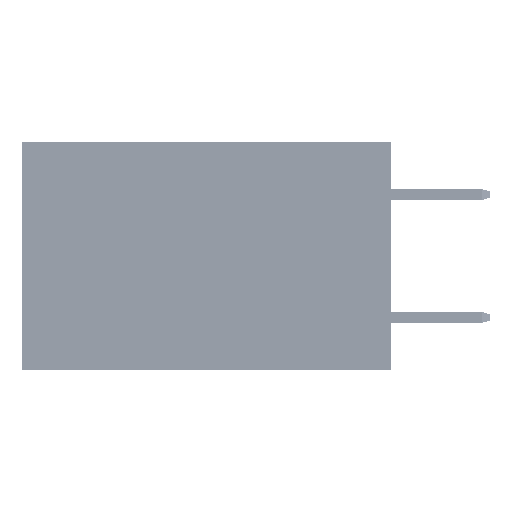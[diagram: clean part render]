
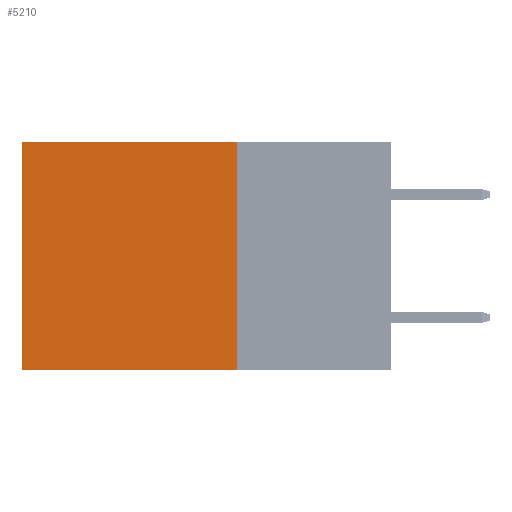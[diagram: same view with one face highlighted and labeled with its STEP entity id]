
A CAD part, left-side view. The second image highlights one B-rep face of the part: STEP entity #5210.
In plain terms, the highlighted planar face has unit normal (-1, 0, 0).
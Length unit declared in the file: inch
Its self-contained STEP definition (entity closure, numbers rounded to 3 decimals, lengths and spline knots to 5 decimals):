
#3151 = CARTESIAN_POINT ( 'NONE',  ( 0.2875, 0.25, 0. ) ) ;
#4904 = VECTOR ( 'NONE', #6634, 39.37008 ) ;
#5210 = ADVANCED_FACE ( 'NONE', ( #14518 ), #25948, .F. ) ;
#5528 = ORIENTED_EDGE ( 'NONE', *, *, #47186, .T. ) ;
#6573 = ORIENTED_EDGE ( 'NONE', *, *, #26342, .F. ) ;
#6634 = DIRECTION ( 'NONE',  ( 0., 1., 0. ) ) ;
#7434 = VERTEX_POINT ( 'NONE', #32129 ) ;
#8522 = VECTOR ( 'NONE', #39454, 39.37008 ) ;
#9106 = ORIENTED_EDGE ( 'NONE', *, *, #10187, .F. ) ;
#9774 = VECTOR ( 'NONE', #40423, 39.37008 ) ;
#10187 = EDGE_CURVE ( 'NONE', #12252, #39724, #34693, .T. ) ;
#10307 = EDGE_CURVE ( 'NONE', #17589, #7434, #33476, .T. ) ;
#12252 = VERTEX_POINT ( 'NONE', #25868 ) ;
#12805 = LINE ( 'NONE', #33045, #9774 ) ;
#14476 = DIRECTION ( 'NONE',  ( 1., 0., 0. ) ) ;
#14518 = FACE_OUTER_BOUND ( 'NONE', #28365, .T. ) ;
#17578 = CARTESIAN_POINT ( 'NONE',  ( 0.2875, 0.25, 0. ) ) ;
#17589 = VERTEX_POINT ( 'NONE', #31021 ) ;
#25868 = CARTESIAN_POINT ( 'NONE',  ( 0.2875, 0.25, -0.37 ) ) ;
#25948 = PLANE ( 'NONE',  #30757 ) ;
#26342 = EDGE_CURVE ( 'NONE', #17589, #12252, #12805, .T. ) ;
#26993 = ORIENTED_EDGE ( 'NONE', *, *, #10307, .T. ) ;
#28257 = CARTESIAN_POINT ( 'NONE',  ( 0.2875, 0.6, -0.37 ) ) ;
#28365 = EDGE_LOOP ( 'NONE', ( #5528, #9106, #6573, #26993 ) ) ;
#29901 = DIRECTION ( 'NONE',  ( 0., 0., -1. ) ) ;
#30757 = AXIS2_PLACEMENT_3D ( 'NONE', #3151, #14476, #29901 ) ;
#31021 = CARTESIAN_POINT ( 'NONE',  ( 0.2875, 0.25, 0. ) ) ;
#31743 = CARTESIAN_POINT ( 'NONE',  ( 0.2875, 0.25, -0.37 ) ) ;
#32129 = CARTESIAN_POINT ( 'NONE',  ( 0.2875, 0.6, 0. ) ) ;
#33045 = CARTESIAN_POINT ( 'NONE',  ( 0.2875, 0.25, 0. ) ) ;
#33476 = LINE ( 'NONE', #17578, #4904 ) ;
#34390 = LINE ( 'NONE', #45089, #36611 ) ;
#34693 = LINE ( 'NONE', #31743, #8522 ) ;
#36611 = VECTOR ( 'NONE', #45919, 39.37008 ) ;
#39454 = DIRECTION ( 'NONE',  ( 0., 1., 0. ) ) ;
#39724 = VERTEX_POINT ( 'NONE', #28257 ) ;
#40423 = DIRECTION ( 'NONE',  ( 0., 0., -1. ) ) ;
#45089 = CARTESIAN_POINT ( 'NONE',  ( 0.2875, 0.6, 0. ) ) ;
#45919 = DIRECTION ( 'NONE',  ( 0., 0., -1. ) ) ;
#47186 = EDGE_CURVE ( 'NONE', #7434, #39724, #34390, .T. ) ;
